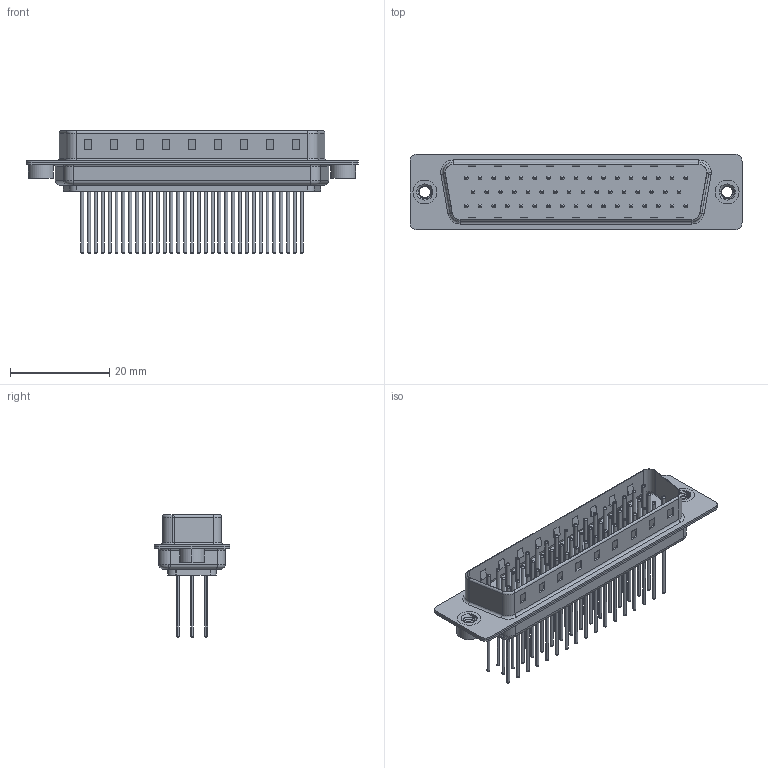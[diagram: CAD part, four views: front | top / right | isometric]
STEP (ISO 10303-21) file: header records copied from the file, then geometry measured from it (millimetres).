
FILE_DESCRIPTION (( 'STEP AP203' ), '1' );
FILE_NAME ('627-M50-223-WN2.STEP', '2020-07-17T17:05:41', ( '' ), ( '' ), 'SwSTEP 2.0', 'SolidWorks 2020', '' );
FILE_SCHEMA (( 'CONFIG_CONTROL_DESIGN' ));
Length unit declared in the file: millimetre
Products named in the file (8): 627M Contact Row 2_23; 627M Shell Rear_50 Contacts; 627M Housing_50 Contacts; 627M Contact Row 3_23; 627M 4-40 Threaded Rivet; 627-M50-223-WN2; 627M Contact Row 1_23; 627M Shell Front_50 Contacts
Assembly tree (55 placements, depth 2):
  627-M50-223-WN2
    627M Housing_50 Contacts
    627M Shell Front_50 Contacts
    627M Shell Rear_50 Contacts
    627M Contact Row 1_23  x17
    627M Contact Row 2_23  x16
    627M Contact Row 3_23  x17
    627M 4-40 Threaded Rivet  x2
Bounding box: 67 x 15.3 x 24.77 mm (x, y, z)
Volume: 4622 mm3; surface area: 11346.7 mm2
Topology: 55 solids, 55 shells, 2262 faces, 4757 edges, 2866 vertices
Faces by surface type: torus 850, cylinder 841, plane 553, cone 12, bspline 6
Entity records: 29260 total; most frequent: CARTESIAN_POINT 5813, DIRECTION 4880, ORIENTED_EDGE 4088, EDGE_CURVE 2044, AXIS2_PLACEMENT_3D 1962, VERTEX_POINT 1310, EDGE_LOOP 1134, CIRCLE 1041
